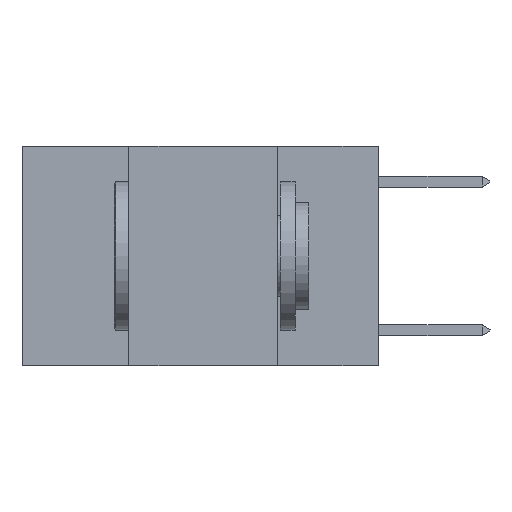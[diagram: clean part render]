
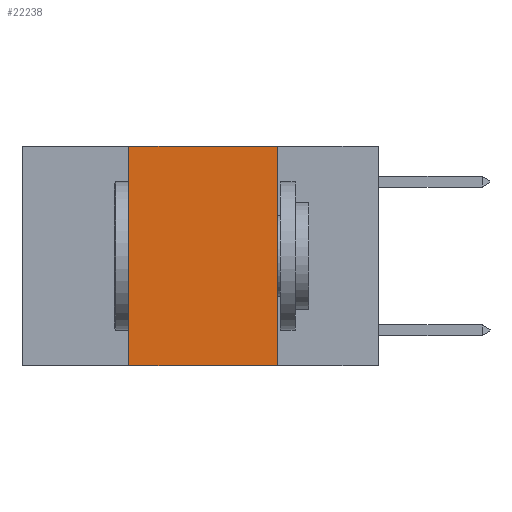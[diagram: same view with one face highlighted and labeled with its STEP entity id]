
A CAD part, left-side view. The second image highlights one B-rep face of the part: STEP entity #22238.
In plain terms, the highlighted planar face has unit normal (-1, 0, 0).
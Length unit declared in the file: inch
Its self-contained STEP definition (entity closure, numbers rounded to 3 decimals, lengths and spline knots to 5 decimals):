
#185 = EDGE_LOOP ( 'NONE', ( #13200, #13702, #16804, #22914 ) ) ;
#193 = VECTOR ( 'NONE', #17716, 39.37008 ) ;
#911 = VERTEX_POINT ( 'NONE', #22922 ) ;
#1744 = CARTESIAN_POINT ( 'NONE',  ( 0., 0.6, 0. ) ) ;
#3086 = CARTESIAN_POINT ( 'NONE',  ( 0., 0.17, -0.37 ) ) ;
#4739 = VERTEX_POINT ( 'NONE', #18915 ) ;
#6004 = EDGE_CURVE ( 'NONE', #911, #19279, #18916, .T. ) ;
#7902 = LINE ( 'NONE', #18873, #17839 ) ;
#9362 = CARTESIAN_POINT ( 'NONE',  ( 0., 0.42, 0. ) ) ;
#9517 = EDGE_CURVE ( 'NONE', #9920, #4739, #19239, .T. ) ;
#9920 = VERTEX_POINT ( 'NONE', #20445 ) ;
#12072 = DIRECTION ( 'NONE',  ( 1., 0., 0. ) ) ;
#13200 = ORIENTED_EDGE ( 'NONE', *, *, #6004, .F. ) ;
#13702 = ORIENTED_EDGE ( 'NONE', *, *, #14673, .F. ) ;
#14357 = CARTESIAN_POINT ( 'NONE',  ( 0., 0.17, 0. ) ) ;
#14673 = EDGE_CURVE ( 'NONE', #4739, #911, #7902, .T. ) ;
#14994 = AXIS2_PLACEMENT_3D ( 'NONE', #1744, #12072, #25567 ) ;
#16483 = LINE ( 'NONE', #25309, #193 ) ;
#16804 = ORIENTED_EDGE ( 'NONE', *, *, #9517, .F. ) ;
#17716 = DIRECTION ( 'NONE',  ( 0., -1., 0. ) ) ;
#17839 = VECTOR ( 'NONE', #22807, 39.37008 ) ;
#17930 = PLANE ( 'NONE',  #14994 ) ;
#17936 = EDGE_CURVE ( 'NONE', #9920, #19279, #16483, .T. ) ;
#18725 = VECTOR ( 'NONE', #24182, 39.37008 ) ;
#18873 = CARTESIAN_POINT ( 'NONE',  ( 0., 0.6, 0. ) ) ;
#18915 = CARTESIAN_POINT ( 'NONE',  ( 0., 0.42, 0. ) ) ;
#18916 = LINE ( 'NONE', #14357, #18725 ) ;
#19185 = DIRECTION ( 'NONE',  ( 0., 0., 1. ) ) ;
#19239 = LINE ( 'NONE', #9362, #19321 ) ;
#19279 = VERTEX_POINT ( 'NONE', #3086 ) ;
#19321 = VECTOR ( 'NONE', #19185, 39.37008 ) ;
#19716 = FACE_OUTER_BOUND ( 'NONE', #185, .T. ) ;
#20445 = CARTESIAN_POINT ( 'NONE',  ( 0., 0.42, -0.37 ) ) ;
#22238 = ADVANCED_FACE ( 'NONE', ( #19716 ), #17930, .F. ) ;
#22807 = DIRECTION ( 'NONE',  ( 0., -1., 0. ) ) ;
#22914 = ORIENTED_EDGE ( 'NONE', *, *, #17936, .T. ) ;
#22922 = CARTESIAN_POINT ( 'NONE',  ( 0., 0.17, 0. ) ) ;
#24182 = DIRECTION ( 'NONE',  ( 0., 0., -1. ) ) ;
#25309 = CARTESIAN_POINT ( 'NONE',  ( 0., 0.6, -0.37 ) ) ;
#25567 = DIRECTION ( 'NONE',  ( 0., 0., -1. ) ) ;
